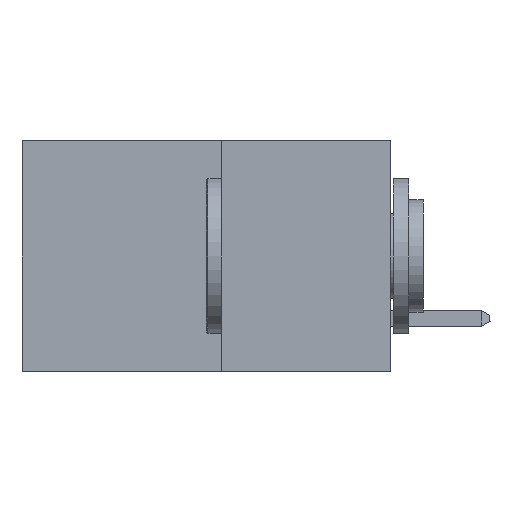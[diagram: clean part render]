
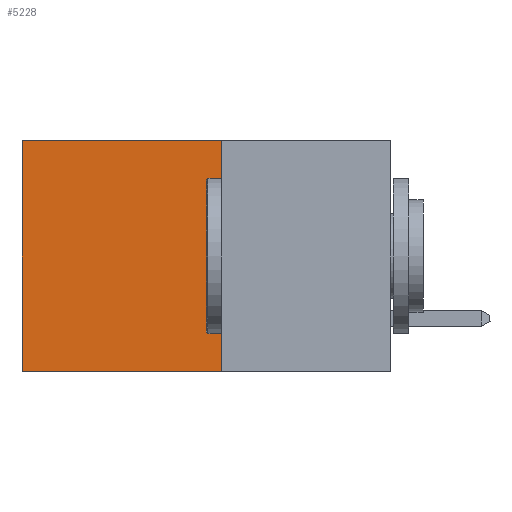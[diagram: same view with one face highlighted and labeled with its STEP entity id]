
A CAD part, left-side view. The second image highlights one B-rep face of the part: STEP entity #5228.
In plain terms, the highlighted planar face has unit normal (-1, 0, 0).
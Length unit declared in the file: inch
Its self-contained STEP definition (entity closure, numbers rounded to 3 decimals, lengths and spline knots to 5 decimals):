
#77 = LINE ( 'NONE', #5564, #8665 ) ;
#247 = DIRECTION ( 'NONE',  ( 0., 1., 0. ) ) ;
#1290 = CARTESIAN_POINT ( 'NONE',  ( 0.277, 0.59, 0. ) ) ;
#1491 = VECTOR ( 'NONE', #12338, 39.37008 ) ;
#1514 = EDGE_CURVE ( 'NONE', #2127, #5068, #10071, .T. ) ;
#1677 = ORIENTED_EDGE ( 'NONE', *, *, #5161, .F. ) ;
#2122 = AXIS2_PLACEMENT_3D ( 'NONE', #10317, #10135, #10107 ) ;
#2127 = VERTEX_POINT ( 'NONE', #1290 ) ;
#2350 = EDGE_LOOP ( 'NONE', ( #5989, #5964, #1677, #8207 ) ) ;
#2582 = VERTEX_POINT ( 'NONE', #9296 ) ;
#2747 = VECTOR ( 'NONE', #11543, 39.37008 ) ;
#3718 = VERTEX_POINT ( 'NONE', #9471 ) ;
#5052 = LINE ( 'NONE', #7764, #7946 ) ;
#5068 = VERTEX_POINT ( 'NONE', #12615 ) ;
#5161 = EDGE_CURVE ( 'NONE', #3718, #2582, #11255, .T. ) ;
#5228 = ADVANCED_FACE ( 'NONE', ( #7779 ), #10260, .F. ) ;
#5564 = CARTESIAN_POINT ( 'NONE',  ( 0.277, 0.27, 0. ) ) ;
#5964 = ORIENTED_EDGE ( 'NONE', *, *, #6104, .F. ) ;
#5989 = ORIENTED_EDGE ( 'NONE', *, *, #1514, .T. ) ;
#6104 = EDGE_CURVE ( 'NONE', #2582, #5068, #5052, .T. ) ;
#7764 = CARTESIAN_POINT ( 'NONE',  ( 0.277, 0.27, -0.37 ) ) ;
#7779 = FACE_OUTER_BOUND ( 'NONE', #2350, .T. ) ;
#7798 = DIRECTION ( 'NONE',  ( 0., 1., 0. ) ) ;
#7946 = VECTOR ( 'NONE', #7798, 39.37008 ) ;
#8207 = ORIENTED_EDGE ( 'NONE', *, *, #11444, .T. ) ;
#8573 = CARTESIAN_POINT ( 'NONE',  ( 0.277, 0.59, -0.37 ) ) ;
#8665 = VECTOR ( 'NONE', #247, 39.37008 ) ;
#9296 = CARTESIAN_POINT ( 'NONE',  ( 0.277, 0.27, -0.37 ) ) ;
#9471 = CARTESIAN_POINT ( 'NONE',  ( 0.277, 0.27, 0. ) ) ;
#10071 = LINE ( 'NONE', #8573, #1491 ) ;
#10107 = DIRECTION ( 'NONE',  ( 0., 0., -1. ) ) ;
#10135 = DIRECTION ( 'NONE',  ( 1., 0., 0. ) ) ;
#10260 = PLANE ( 'NONE',  #2122 ) ;
#10317 = CARTESIAN_POINT ( 'NONE',  ( 0.277, 0.27, -0.37 ) ) ;
#11255 = LINE ( 'NONE', #11631, #2747 ) ;
#11444 = EDGE_CURVE ( 'NONE', #3718, #2127, #77, .T. ) ;
#11543 = DIRECTION ( 'NONE',  ( 0., 0., -1. ) ) ;
#11631 = CARTESIAN_POINT ( 'NONE',  ( 0.277, 0.27, -0.37 ) ) ;
#12338 = DIRECTION ( 'NONE',  ( 0., 0., -1. ) ) ;
#12615 = CARTESIAN_POINT ( 'NONE',  ( 0.277, 0.59, -0.37 ) ) ;
